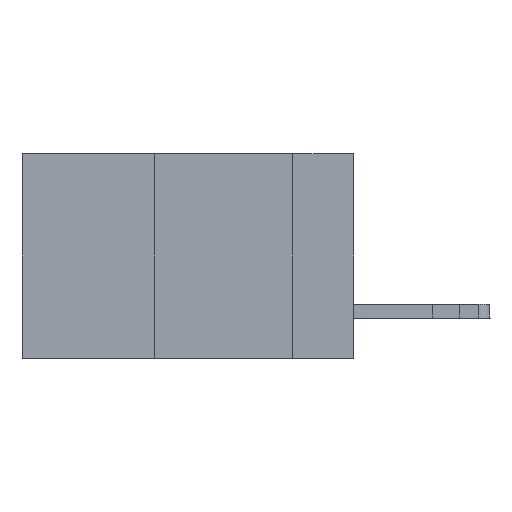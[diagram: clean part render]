
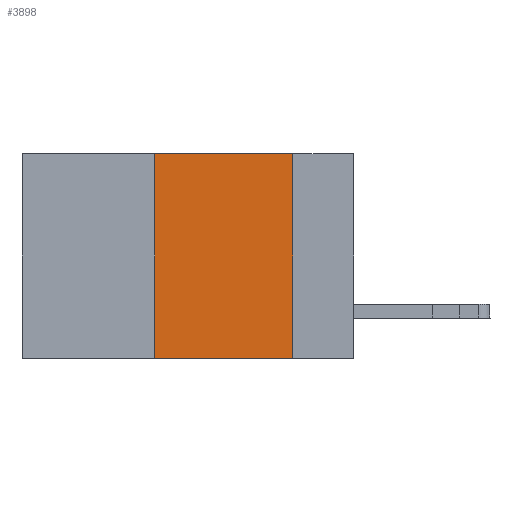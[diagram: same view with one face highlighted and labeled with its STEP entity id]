
A CAD part, left-side view. The second image highlights one B-rep face of the part: STEP entity #3898.
In plain terms, the highlighted planar face has unit normal (-1, 0, 0).
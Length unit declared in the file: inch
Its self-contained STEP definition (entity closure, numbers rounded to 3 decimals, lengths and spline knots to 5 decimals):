
#484 = LINE ( 'NONE', #14693, #12963 ) ;
#972 = ORIENTED_EDGE ( 'NONE', *, *, #7993, .F. ) ;
#1183 = ORIENTED_EDGE ( 'NONE', *, *, #3764, .T. ) ;
#1373 = ORIENTED_EDGE ( 'NONE', *, *, #5602, .F. ) ;
#1546 = VERTEX_POINT ( 'NONE', #13191 ) ;
#2006 = LINE ( 'NONE', #2716, #8105 ) ;
#2612 = CARTESIAN_POINT ( 'NONE',  ( 0., 0.36, 0. ) ) ;
#2716 = CARTESIAN_POINT ( 'NONE',  ( 0., 0.11, 0. ) ) ;
#3764 = EDGE_CURVE ( 'NONE', #1546, #10334, #8042, .T. ) ;
#3887 = AXIS2_PLACEMENT_3D ( 'NONE', #8603, #8559, #8539 ) ;
#3898 = ADVANCED_FACE ( 'NONE', ( #12452 ), #8615, .F. ) ;
#5602 = EDGE_CURVE ( 'NONE', #8341, #7294, #484, .T. ) ;
#5723 = VECTOR ( 'NONE', #14563, 39.37008 ) ;
#7294 = VERTEX_POINT ( 'NONE', #13345 ) ;
#7993 = EDGE_CURVE ( 'NONE', #7294, #10334, #2006, .T. ) ;
#8042 = LINE ( 'NONE', #10069, #13925 ) ;
#8105 = VECTOR ( 'NONE', #13485, 39.37008 ) ;
#8341 = VERTEX_POINT ( 'NONE', #2612 ) ;
#8539 = DIRECTION ( 'NONE',  ( 0., 0., -1. ) ) ;
#8559 = DIRECTION ( 'NONE',  ( 1., 0., 0. ) ) ;
#8603 = CARTESIAN_POINT ( 'NONE',  ( 0., 0.6, 0. ) ) ;
#8615 = PLANE ( 'NONE',  #3887 ) ;
#8849 = DIRECTION ( 'NONE',  ( 0., -1., 0. ) ) ;
#9622 = EDGE_LOOP ( 'NONE', ( #972, #1373, #9763, #1183 ) ) ;
#9763 = ORIENTED_EDGE ( 'NONE', *, *, #14725, .F. ) ;
#9966 = DIRECTION ( 'NONE',  ( 0., -1., 0. ) ) ;
#10069 = CARTESIAN_POINT ( 'NONE',  ( 0., 0.6, -0.37 ) ) ;
#10334 = VERTEX_POINT ( 'NONE', #12412 ) ;
#12412 = CARTESIAN_POINT ( 'NONE',  ( 0., 0.11, -0.37 ) ) ;
#12452 = FACE_OUTER_BOUND ( 'NONE', #9622, .T. ) ;
#12963 = VECTOR ( 'NONE', #8849, 39.37008 ) ;
#13191 = CARTESIAN_POINT ( 'NONE',  ( 0., 0.36, -0.37 ) ) ;
#13345 = CARTESIAN_POINT ( 'NONE',  ( 0., 0.11, 0. ) ) ;
#13372 = CARTESIAN_POINT ( 'NONE',  ( 0., 0.36, 0. ) ) ;
#13485 = DIRECTION ( 'NONE',  ( 0., 0., -1. ) ) ;
#13925 = VECTOR ( 'NONE', #9966, 39.37008 ) ;
#14563 = DIRECTION ( 'NONE',  ( 0., 0., 1. ) ) ;
#14693 = CARTESIAN_POINT ( 'NONE',  ( 0., 0.6, 0. ) ) ;
#14725 = EDGE_CURVE ( 'NONE', #1546, #8341, #15139, .T. ) ;
#15139 = LINE ( 'NONE', #13372, #5723 ) ;
